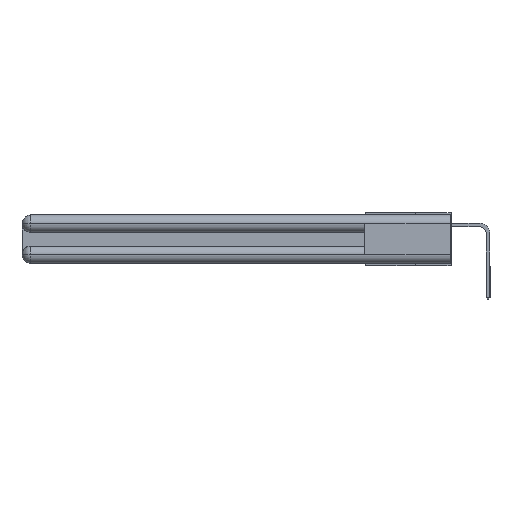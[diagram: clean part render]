
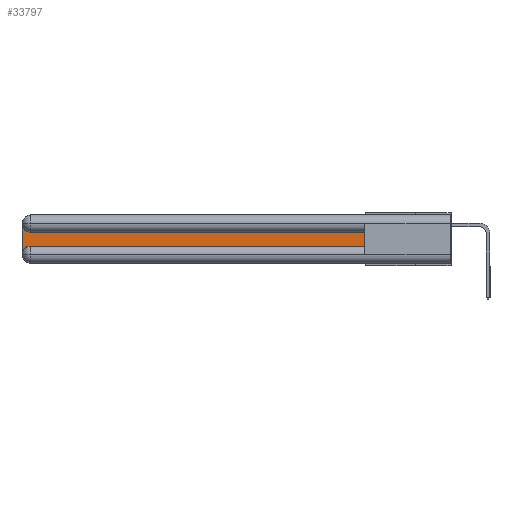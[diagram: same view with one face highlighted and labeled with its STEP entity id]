
A CAD part, left-side view. The second image highlights one B-rep face of the part: STEP entity #33797.
In plain terms, the highlighted planar face has unit normal (-1, 0, 0).
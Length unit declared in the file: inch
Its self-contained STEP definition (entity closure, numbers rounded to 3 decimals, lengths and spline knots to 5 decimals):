
#317 = ORIENTED_EDGE ( 'NONE', *, *, #10387, .T. ) ;
#2062 = VERTEX_POINT ( 'NONE', #11886 ) ;
#2970 = DIRECTION ( 'NONE',  ( 0., 0., -1. ) ) ;
#3869 = LINE ( 'NONE', #13807, #30909 ) ;
#4156 = ORIENTED_EDGE ( 'NONE', *, *, #14929, .T. ) ;
#4861 = CARTESIAN_POINT ( 'NONE',  ( 0.075, 2.94, -0.0625 ) ) ;
#5699 = CARTESIAN_POINT ( 'NONE',  ( 0.075, 3., -0.1225 ) ) ;
#6234 = CARTESIAN_POINT ( 'NONE',  ( 0.075, 3., -0.0625 ) ) ;
#6602 = ORIENTED_EDGE ( 'NONE', *, *, #25035, .T. ) ;
#7107 = DIRECTION ( 'NONE',  ( 0., 0., -1. ) ) ;
#8090 = DIRECTION ( 'NONE',  ( 0., 1., 0. ) ) ;
#8248 = CIRCLE ( 'NONE', #25601, 0.06 ) ;
#8973 = CARTESIAN_POINT ( 'NONE',  ( 0.075, 3., -0.2175 ) ) ;
#10169 = VERTEX_POINT ( 'NONE', #24911 ) ;
#10387 = EDGE_CURVE ( 'NONE', #19753, #22683, #13134, .T. ) ;
#10497 = AXIS2_PLACEMENT_3D ( 'NONE', #5699, #24159, #2970 ) ;
#11157 = ORIENTED_EDGE ( 'NONE', *, *, #19996, .T. ) ;
#11886 = CARTESIAN_POINT ( 'NONE',  ( 0.075, 0.6, -0.2175 ) ) ;
#12436 = EDGE_LOOP ( 'NONE', ( #4156, #317, #24784, #6602, #33345, #11157 ) ) ;
#12737 = DIRECTION ( 'NONE',  ( 1., 0., 0. ) ) ;
#13134 = CIRCLE ( 'NONE', #32164, 0.06 ) ;
#13807 = CARTESIAN_POINT ( 'NONE',  ( 0.075, 0.6, -0.2175 ) ) ;
#14050 = EDGE_CURVE ( 'NONE', #24564, #2062, #3869, .T. ) ;
#14929 = EDGE_CURVE ( 'NONE', #15195, #19753, #21475, .T. ) ;
#14998 = VECTOR ( 'NONE', #16917, 39.37008 ) ;
#15195 = VERTEX_POINT ( 'NONE', #22180 ) ;
#15423 = DIRECTION ( 'NONE',  ( 0., -1., 0. ) ) ;
#16917 = DIRECTION ( 'NONE',  ( 0., 0., -1. ) ) ;
#17562 = CARTESIAN_POINT ( 'NONE',  ( 0.075, 2.94, -0.2175 ) ) ;
#18782 = FACE_OUTER_BOUND ( 'NONE', #12436, .T. ) ;
#18785 = PLANE ( 'NONE',  #10497 ) ;
#19556 = LINE ( 'NONE', #8973, #14998 ) ;
#19753 = VERTEX_POINT ( 'NONE', #25692 ) ;
#19996 = EDGE_CURVE ( 'NONE', #2062, #15195, #23797, .T. ) ;
#21475 = LINE ( 'NONE', #33870, #32135 ) ;
#22180 = CARTESIAN_POINT ( 'NONE',  ( 0.075, 0.6, -0.1225 ) ) ;
#22192 = EDGE_CURVE ( 'NONE', #22683, #10169, #19556, .T. ) ;
#22683 = VERTEX_POINT ( 'NONE', #6234 ) ;
#22824 = CARTESIAN_POINT ( 'NONE',  ( 0.075, 2.94, -0.2775 ) ) ;
#23171 = DIRECTION ( 'NONE',  ( 0., 0., -1. ) ) ;
#23797 = LINE ( 'NONE', #26996, #33577 ) ;
#24159 = DIRECTION ( 'NONE',  ( 1., 0., 0. ) ) ;
#24564 = VERTEX_POINT ( 'NONE', #17562 ) ;
#24649 = DIRECTION ( 'NONE',  ( 0., 0., 1. ) ) ;
#24784 = ORIENTED_EDGE ( 'NONE', *, *, #22192, .T. ) ;
#24911 = CARTESIAN_POINT ( 'NONE',  ( 0.075, 3., -0.2775 ) ) ;
#25035 = EDGE_CURVE ( 'NONE', #10169, #24564, #8248, .T. ) ;
#25601 = AXIS2_PLACEMENT_3D ( 'NONE', #22824, #27967, #7107 ) ;
#25692 = CARTESIAN_POINT ( 'NONE',  ( 0.075, 2.94, -0.1225 ) ) ;
#26996 = CARTESIAN_POINT ( 'NONE',  ( 0.075, 0.6, -0.2175 ) ) ;
#27967 = DIRECTION ( 'NONE',  ( 1., 0., 0. ) ) ;
#30909 = VECTOR ( 'NONE', #15423, 39.37008 ) ;
#32135 = VECTOR ( 'NONE', #8090, 39.37008 ) ;
#32164 = AXIS2_PLACEMENT_3D ( 'NONE', #4861, #12737, #23171 ) ;
#33345 = ORIENTED_EDGE ( 'NONE', *, *, #14050, .T. ) ;
#33577 = VECTOR ( 'NONE', #24649, 39.37008 ) ;
#33797 = ADVANCED_FACE ( 'NONE', ( #18782 ), #18785, .F. ) ;
#33870 = CARTESIAN_POINT ( 'NONE',  ( 0.075, 0.6, -0.1225 ) ) ;
